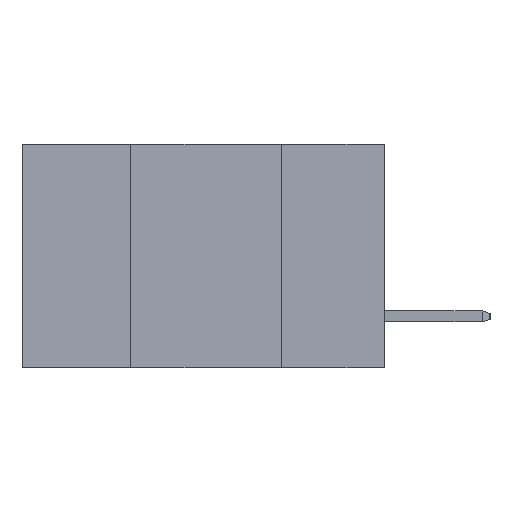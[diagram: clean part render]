
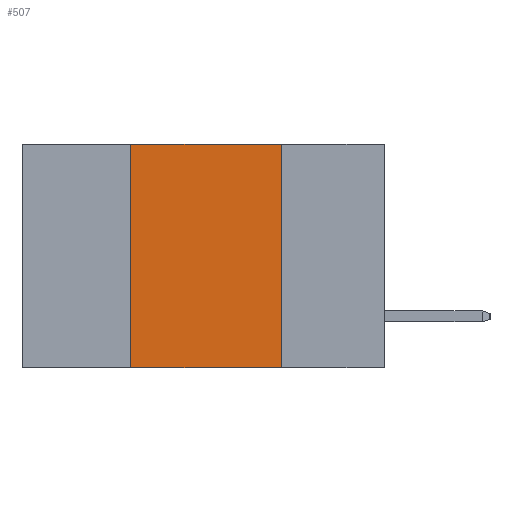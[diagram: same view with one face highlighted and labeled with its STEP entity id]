
A CAD part, left-side view. The second image highlights one B-rep face of the part: STEP entity #507.
In plain terms, the highlighted planar face has unit normal (-1, 0, 0).
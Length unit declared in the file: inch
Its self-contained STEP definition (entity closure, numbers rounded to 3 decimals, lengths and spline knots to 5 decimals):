
#69 = DIRECTION ( 'NONE',  ( 0., -1., 0. ) ) ;
#486 = VECTOR ( 'NONE', #11191, 39.37008 ) ;
#507 = ADVANCED_FACE ( 'NONE', ( #8371 ), #3940, .F. ) ;
#682 = CARTESIAN_POINT ( 'NONE',  ( 0., 0.42, 0. ) ) ;
#2145 = CARTESIAN_POINT ( 'NONE',  ( 0., 0.6, 0. ) ) ;
#2242 = CARTESIAN_POINT ( 'NONE',  ( 0., 0.42, -0.37 ) ) ;
#2636 = EDGE_CURVE ( 'NONE', #6825, #6029, #5663, .T. ) ;
#2687 = VECTOR ( 'NONE', #7462, 39.37008 ) ;
#2882 = EDGE_CURVE ( 'NONE', #6825, #10866, #5513, .T. ) ;
#3571 = CARTESIAN_POINT ( 'NONE',  ( 0., 0.17, -0.37 ) ) ;
#3604 = EDGE_CURVE ( 'NONE', #6029, #9534, #4483, .T. ) ;
#3651 = ORIENTED_EDGE ( 'NONE', *, *, #5777, .F. ) ;
#3813 = ORIENTED_EDGE ( 'NONE', *, *, #3604, .F. ) ;
#3940 = PLANE ( 'NONE',  #5365 ) ;
#4023 = DIRECTION ( 'NONE',  ( 0., 0., -1. ) ) ;
#4155 = CARTESIAN_POINT ( 'NONE',  ( 0., 0.17, 0. ) ) ;
#4218 = ORIENTED_EDGE ( 'NONE', *, *, #2636, .F. ) ;
#4483 = LINE ( 'NONE', #2145, #11302 ) ;
#4512 = ORIENTED_EDGE ( 'NONE', *, *, #2882, .T. ) ;
#4654 = DIRECTION ( 'NONE',  ( 0., 0., 1. ) ) ;
#5151 = EDGE_LOOP ( 'NONE', ( #3651, #3813, #4218, #4512 ) ) ;
#5365 = AXIS2_PLACEMENT_3D ( 'NONE', #6888, #7577, #4023 ) ;
#5513 = LINE ( 'NONE', #11252, #486 ) ;
#5663 = LINE ( 'NONE', #9035, #8332 ) ;
#5777 = EDGE_CURVE ( 'NONE', #9534, #10866, #7315, .T. ) ;
#6029 = VERTEX_POINT ( 'NONE', #682 ) ;
#6825 = VERTEX_POINT ( 'NONE', #2242 ) ;
#6888 = CARTESIAN_POINT ( 'NONE',  ( 0., 0.6, 0. ) ) ;
#7315 = LINE ( 'NONE', #10141, #2687 ) ;
#7462 = DIRECTION ( 'NONE',  ( 0., 0., -1. ) ) ;
#7577 = DIRECTION ( 'NONE',  ( 1., 0., 0. ) ) ;
#8332 = VECTOR ( 'NONE', #4654, 39.37008 ) ;
#8371 = FACE_OUTER_BOUND ( 'NONE', #5151, .T. ) ;
#9035 = CARTESIAN_POINT ( 'NONE',  ( 0., 0.42, 0. ) ) ;
#9534 = VERTEX_POINT ( 'NONE', #4155 ) ;
#10141 = CARTESIAN_POINT ( 'NONE',  ( 0., 0.17, 0. ) ) ;
#10866 = VERTEX_POINT ( 'NONE', #3571 ) ;
#11191 = DIRECTION ( 'NONE',  ( 0., -1., 0. ) ) ;
#11252 = CARTESIAN_POINT ( 'NONE',  ( 0., 0.6, -0.37 ) ) ;
#11302 = VECTOR ( 'NONE', #69, 39.37008 ) ;
